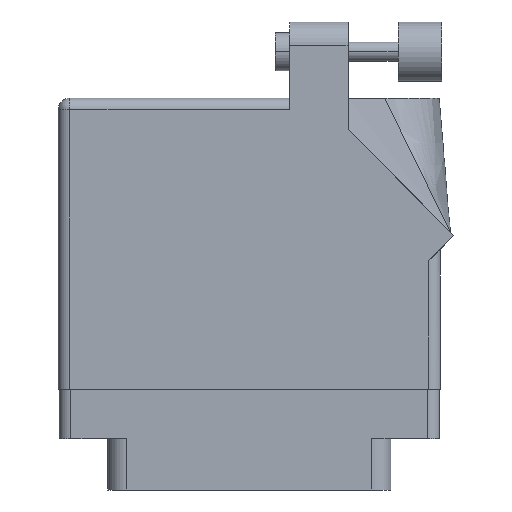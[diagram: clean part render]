
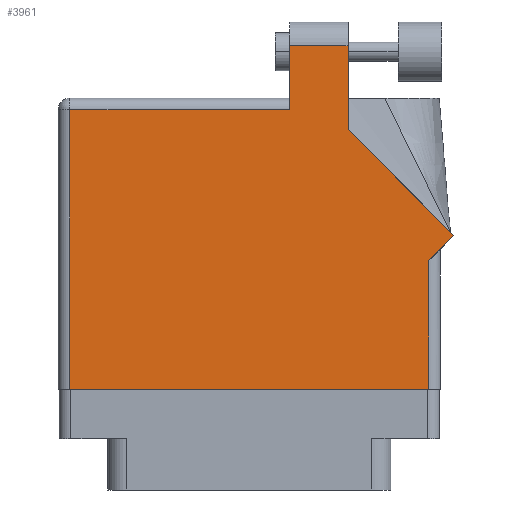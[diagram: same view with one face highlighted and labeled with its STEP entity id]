
A CAD part, front view. The second image highlights one B-rep face of the part: STEP entity #3961.
In plain terms, the highlighted face is planar.
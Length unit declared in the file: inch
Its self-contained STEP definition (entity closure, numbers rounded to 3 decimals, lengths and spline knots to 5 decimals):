
#119 = CARTESIAN_POINT ( 'NONE',  ( 0., 0., 0. ) ) ;
#627 = EDGE_CURVE ( 'NONE', #30402, #16951, #10634, .T. ) ;
#674 = DIRECTION ( 'NONE',  ( -1., 0., 0. ) ) ;
#753 = VERTEX_POINT ( 'NONE', #31274 ) ;
#887 = EDGE_CURVE ( 'NONE', #8640, #30402, #18651, .T. ) ;
#1991 = ORIENTED_EDGE ( 'NONE', *, *, #29911, .T. ) ;
#2440 = DIRECTION ( 'NONE',  ( 0., 1., 0. ) ) ;
#2735 = EDGE_CURVE ( 'NONE', #18068, #753, #7107, .T. ) ;
#3449 = VECTOR ( 'NONE', #30591, 39.37008 ) ;
#3874 = LINE ( 'NONE', #21717, #28315 ) ;
#3961 = ADVANCED_FACE ( 'NONE', ( #12543 ), #6234, .F. ) ;
#4600 = CARTESIAN_POINT ( 'NONE',  ( 0.062, 0., 0. ) ) ;
#5299 = CARTESIAN_POINT ( 'NONE',  ( 1.524, 1.36442, 0. ) ) ;
#6112 = CARTESIAN_POINT ( 'NONE',  ( 0., 1.53, 0. ) ) ;
#6234 = PLANE ( 'NONE',  #9832 ) ;
#6269 = VECTOR ( 'NONE', #2440, 39.37008 ) ;
#6273 = EDGE_LOOP ( 'NONE', ( #24197, #1991, #21358, #26523, #12251, #30251, #17355, #29700, #33922 ) ) ;
#6934 = VERTEX_POINT ( 'NONE', #32804 ) ;
#7107 = LINE ( 'NONE', #21340, #26525 ) ;
#7644 = CARTESIAN_POINT ( 'NONE',  ( 1.524, 1.805, 0. ) ) ;
#7675 = DIRECTION ( 'NONE',  ( 0., -1., 0. ) ) ;
#8176 = VERTEX_POINT ( 'NONE', #5299 ) ;
#8485 = CARTESIAN_POINT ( 'NONE',  ( 1.948, 0., 0. ) ) ;
#8640 = VERTEX_POINT ( 'NONE', #4600 ) ;
#9066 = VECTOR ( 'NONE', #16971, 39.37008 ) ;
#9245 = CARTESIAN_POINT ( 'NONE',  ( 1.217, 1.805, 0. ) ) ;
#9832 = AXIS2_PLACEMENT_3D ( 'NONE', #6112, #19346, #674 ) ;
#10634 = LINE ( 'NONE', #27875, #3449 ) ;
#11216 = EDGE_CURVE ( 'NONE', #6934, #8176, #24431, .T. ) ;
#11371 = CARTESIAN_POINT ( 'NONE',  ( 1.217, 1.805, 0. ) ) ;
#12251 = ORIENTED_EDGE ( 'NONE', *, *, #15965, .T. ) ;
#12543 = FACE_OUTER_BOUND ( 'NONE', #6273, .T. ) ;
#13201 = CARTESIAN_POINT ( 'NONE',  ( 1.524, 1.36442, 0. ) ) ;
#14389 = VECTOR ( 'NONE', #29565, 39.37008 ) ;
#15249 = VERTEX_POINT ( 'NONE', #20357 ) ;
#15965 = EDGE_CURVE ( 'NONE', #15249, #8640, #3874, .T. ) ;
#16821 = LINE ( 'NONE', #13201, #6269 ) ;
#16951 = VERTEX_POINT ( 'NONE', #19989 ) ;
#16971 = DIRECTION ( 'NONE',  ( -1., 0., 0. ) ) ;
#17355 = ORIENTED_EDGE ( 'NONE', *, *, #627, .T. ) ;
#18068 = VERTEX_POINT ( 'NONE', #9245 ) ;
#18466 = VERTEX_POINT ( 'NONE', #7644 ) ;
#18605 = CARTESIAN_POINT ( 'NONE',  ( 2.01, 0.737, 0. ) ) ;
#18651 = LINE ( 'NONE', #119, #14389 ) ;
#19346 = DIRECTION ( 'NONE',  ( 0., 0., -1. ) ) ;
#19989 = CARTESIAN_POINT ( 'NONE',  ( 1.948, 0.675, 0. ) ) ;
#20357 = CARTESIAN_POINT ( 'NONE',  ( 0.062, 1.468, 0. ) ) ;
#20786 = LINE ( 'NONE', #18605, #29184 ) ;
#21340 = CARTESIAN_POINT ( 'NONE',  ( 1.217, 1.53, 0. ) ) ;
#21358 = ORIENTED_EDGE ( 'NONE', *, *, #2735, .T. ) ;
#21551 = DIRECTION ( 'NONE',  ( -0.707, 0.707, 0. ) ) ;
#21717 = CARTESIAN_POINT ( 'NONE',  ( 0.062, 0., 0. ) ) ;
#22556 = LINE ( 'NONE', #33430, #9066 ) ;
#23171 = VECTOR ( 'NONE', #21551, 39.37008 ) ;
#24197 = ORIENTED_EDGE ( 'NONE', *, *, #28587, .T. ) ;
#24431 = LINE ( 'NONE', #27087, #23171 ) ;
#24904 = EDGE_CURVE ( 'NONE', #753, #15249, #22556, .T. ) ;
#26426 = VECTOR ( 'NONE', #30174, 39.37008 ) ;
#26523 = ORIENTED_EDGE ( 'NONE', *, *, #24904, .T. ) ;
#26525 = VECTOR ( 'NONE', #7675, 39.37008 ) ;
#27087 = CARTESIAN_POINT ( 'NONE',  ( 2.08071, 0.80771, 0. ) ) ;
#27875 = CARTESIAN_POINT ( 'NONE',  ( 1.948, 0.737, 0. ) ) ;
#28315 = VECTOR ( 'NONE', #29699, 39.37008 ) ;
#28587 = EDGE_CURVE ( 'NONE', #8176, #18466, #16821, .T. ) ;
#29184 = VECTOR ( 'NONE', #34363, 39.37008 ) ;
#29565 = DIRECTION ( 'NONE',  ( 1., 0., 0. ) ) ;
#29699 = DIRECTION ( 'NONE',  ( 0., -1., 0. ) ) ;
#29700 = ORIENTED_EDGE ( 'NONE', *, *, #31844, .T. ) ;
#29911 = EDGE_CURVE ( 'NONE', #18466, #18068, #32680, .T. ) ;
#30174 = DIRECTION ( 'NONE',  ( -1., 0., 0. ) ) ;
#30251 = ORIENTED_EDGE ( 'NONE', *, *, #887, .T. ) ;
#30402 = VERTEX_POINT ( 'NONE', #8485 ) ;
#30591 = DIRECTION ( 'NONE',  ( 0., 1., 0. ) ) ;
#31274 = CARTESIAN_POINT ( 'NONE',  ( 1.217, 1.468, 0. ) ) ;
#31844 = EDGE_CURVE ( 'NONE', #16951, #6934, #20786, .T. ) ;
#32680 = LINE ( 'NONE', #11371, #26426 ) ;
#32804 = CARTESIAN_POINT ( 'NONE',  ( 2.08071, 0.80771, 0. ) ) ;
#33430 = CARTESIAN_POINT ( 'NONE',  ( 0., 1.468, 0. ) ) ;
#33922 = ORIENTED_EDGE ( 'NONE', *, *, #11216, .T. ) ;
#34363 = DIRECTION ( 'NONE',  ( 0.707, 0.707, 0. ) ) ;
